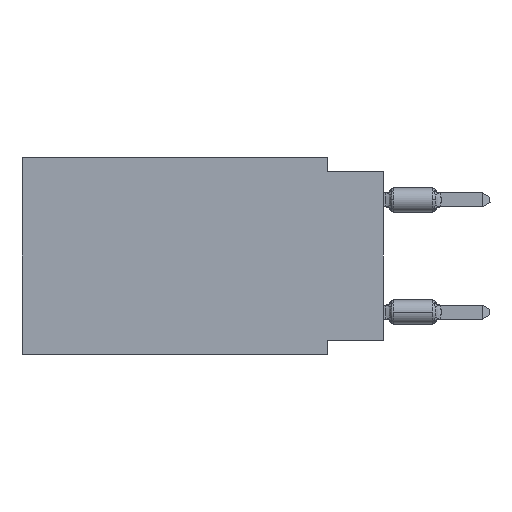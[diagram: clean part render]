
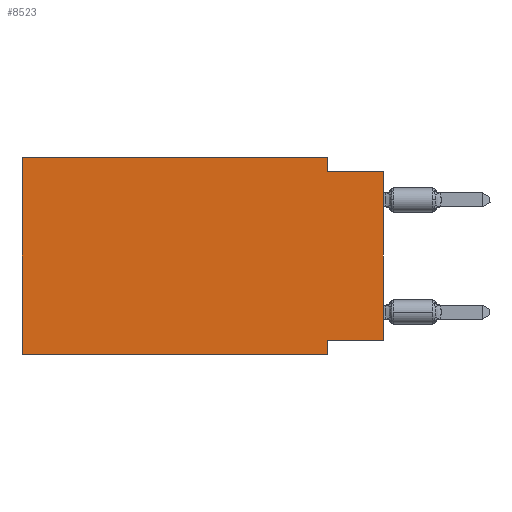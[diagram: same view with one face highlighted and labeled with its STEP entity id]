
A CAD part, left-side view. The second image highlights one B-rep face of the part: STEP entity #8523.
In plain terms, the highlighted planar face has unit normal (-1, 0, 0).
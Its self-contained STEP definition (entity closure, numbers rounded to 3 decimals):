
#3213 = CARTESIAN_POINT ( 'NONE',  ( 0., 16.383, -8.89 ) ) ;
#6265 = ORIENTED_EDGE ( 'NONE', *, *, #28322, .F. ) ;
#8036 = VERTEX_POINT ( 'NONE', #22856 ) ;
#8523 = ADVANCED_FACE ( 'NONE', ( #19941 ), #46300, .F. ) ;
#9229 = DIRECTION ( 'NONE',  ( 1., 0., 0. ) ) ;
#9234 = DIRECTION ( 'NONE',  ( 0., 0., 1. ) ) ;
#9343 = CARTESIAN_POINT ( 'NONE',  ( 0., 2.54, -8.89 ) ) ;
#10510 = CARTESIAN_POINT ( 'NONE',  ( 0., 0., 0. ) ) ;
#12261 = CARTESIAN_POINT ( 'NONE',  ( 0., 2.54, -8.255 ) ) ;
#12321 = VECTOR ( 'NONE', #17738, 1000. ) ;
#13434 = VERTEX_POINT ( 'NONE', #32943 ) ;
#14987 = EDGE_CURVE ( 'NONE', #42404, #8036, #41665, .T. ) ;
#16228 = VERTEX_POINT ( 'NONE', #25032 ) ;
#17082 = DIRECTION ( 'NONE',  ( 0., -1., 0. ) ) ;
#17376 = LINE ( 'NONE', #33438, #12321 ) ;
#17738 = DIRECTION ( 'NONE',  ( 0., 0., -1. ) ) ;
#17831 = CARTESIAN_POINT ( 'NONE',  ( 0., 16.383, -8.89 ) ) ;
#18588 = VECTOR ( 'NONE', #17082, 1000. ) ;
#19941 = FACE_OUTER_BOUND ( 'NONE', #67386, .T. ) ;
#20412 = DIRECTION ( 'NONE',  ( 0., 0., -1. ) ) ;
#21299 = AXIS2_PLACEMENT_3D ( 'NONE', #29914, #9229, #40962 ) ;
#21905 = LINE ( 'NONE', #54320, #46156 ) ;
#22856 = CARTESIAN_POINT ( 'NONE',  ( 0., 16.383, 0. ) ) ;
#23524 = LINE ( 'NONE', #17831, #35313 ) ;
#24032 = EDGE_CURVE ( 'NONE', #42404, #27197, #23524, .T. ) ;
#25032 = CARTESIAN_POINT ( 'NONE',  ( 0., 2.54, 0. ) ) ;
#26896 = DIRECTION ( 'NONE',  ( 0., -1., 0. ) ) ;
#27197 = VERTEX_POINT ( 'NONE', #43338 ) ;
#28322 = EDGE_CURVE ( 'NONE', #16228, #35063, #17376, .T. ) ;
#29879 = ORIENTED_EDGE ( 'NONE', *, *, #45528, .F. ) ;
#29914 = CARTESIAN_POINT ( 'NONE',  ( 0., 16.383, 0. ) ) ;
#32640 = LINE ( 'NONE', #10510, #41764 ) ;
#32943 = CARTESIAN_POINT ( 'NONE',  ( 0., 0., -8.255 ) ) ;
#33438 = CARTESIAN_POINT ( 'NONE',  ( 0., 2.54, 0. ) ) ;
#35063 = VERTEX_POINT ( 'NONE', #51441 ) ;
#35313 = VECTOR ( 'NONE', #50592, 1000. ) ;
#37994 = VECTOR ( 'NONE', #20412, 1000. ) ;
#38632 = ORIENTED_EDGE ( 'NONE', *, *, #42070, .T. ) ;
#38909 = DIRECTION ( 'NONE',  ( 0., 1., 0. ) ) ;
#40962 = DIRECTION ( 'NONE',  ( 0., 0., -1. ) ) ;
#41665 = LINE ( 'NONE', #64467, #69488 ) ;
#41764 = VECTOR ( 'NONE', #43670, 1000. ) ;
#42070 = EDGE_CURVE ( 'NONE', #13434, #61869, #32640, .T. ) ;
#42404 = VERTEX_POINT ( 'NONE', #3213 ) ;
#42940 = ORIENTED_EDGE ( 'NONE', *, *, #24032, .T. ) ;
#43338 = CARTESIAN_POINT ( 'NONE',  ( 0., 2.54, -8.89 ) ) ;
#43670 = DIRECTION ( 'NONE',  ( 0., 0., 1. ) ) ;
#43944 = ORIENTED_EDGE ( 'NONE', *, *, #66121, .F. ) ;
#44592 = EDGE_CURVE ( 'NONE', #8036, #16228, #64858, .T. ) ;
#45528 = EDGE_CURVE ( 'NONE', #13434, #54420, #60326, .T. ) ;
#46156 = VECTOR ( 'NONE', #26896, 1000. ) ;
#46300 = PLANE ( 'NONE',  #21299 ) ;
#47826 = LINE ( 'NONE', #9343, #37994 ) ;
#48617 = ORIENTED_EDGE ( 'NONE', *, *, #44592, .F. ) ;
#49904 = EDGE_CURVE ( 'NONE', #54420, #27197, #47826, .T. ) ;
#50592 = DIRECTION ( 'NONE',  ( 0., -1., 0. ) ) ;
#51441 = CARTESIAN_POINT ( 'NONE',  ( 0., 2.54, -0.635 ) ) ;
#52496 = ORIENTED_EDGE ( 'NONE', *, *, #14987, .F. ) ;
#54320 = CARTESIAN_POINT ( 'NONE',  ( 0., 0., -0.635 ) ) ;
#54420 = VERTEX_POINT ( 'NONE', #12261 ) ;
#55106 = VECTOR ( 'NONE', #38909, 1000. ) ;
#60326 = LINE ( 'NONE', #61715, #55106 ) ;
#61715 = CARTESIAN_POINT ( 'NONE',  ( 0., 0., -8.255 ) ) ;
#61869 = VERTEX_POINT ( 'NONE', #62286 ) ;
#62286 = CARTESIAN_POINT ( 'NONE',  ( 0., 0., -0.635 ) ) ;
#64171 = ORIENTED_EDGE ( 'NONE', *, *, #49904, .F. ) ;
#64467 = CARTESIAN_POINT ( 'NONE',  ( 0., 16.383, 0. ) ) ;
#64858 = LINE ( 'NONE', #66268, #18588 ) ;
#66121 = EDGE_CURVE ( 'NONE', #35063, #61869, #21905, .T. ) ;
#66268 = CARTESIAN_POINT ( 'NONE',  ( 0., 16.383, 0. ) ) ;
#67386 = EDGE_LOOP ( 'NONE', ( #38632, #43944, #6265, #48617, #52496, #42940, #64171, #29879 ) ) ;
#69488 = VECTOR ( 'NONE', #9234, 1000. ) ;
